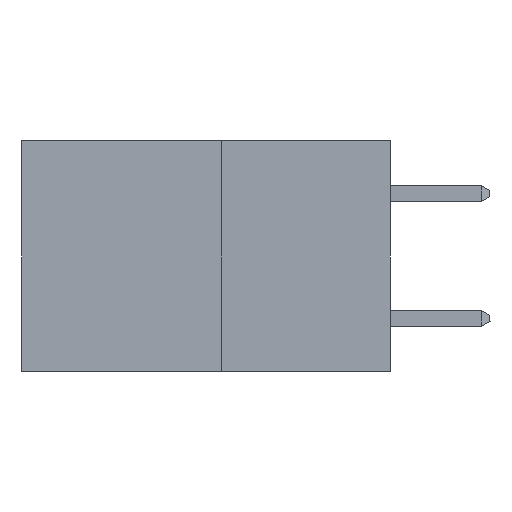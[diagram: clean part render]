
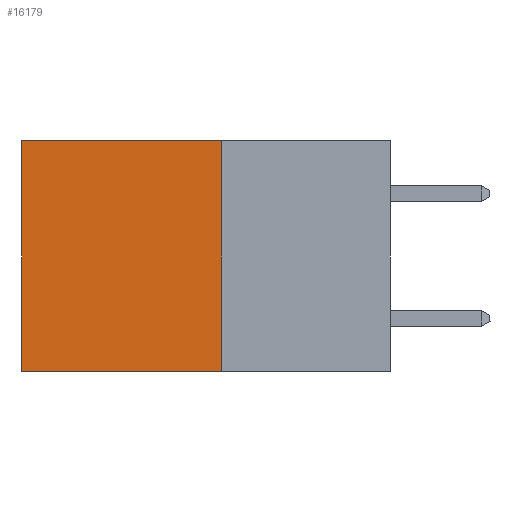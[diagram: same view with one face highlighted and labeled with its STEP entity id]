
A CAD part, left-side view. The second image highlights one B-rep face of the part: STEP entity #16179.
In plain terms, the highlighted planar face has unit normal (-1, 0, 0).
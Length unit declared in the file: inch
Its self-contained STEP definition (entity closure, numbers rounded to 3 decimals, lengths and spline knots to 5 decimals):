
#181 = VERTEX_POINT ( 'NONE', #3201 ) ;
#995 = EDGE_LOOP ( 'NONE', ( #20365, #12897, #12182, #19189 ) ) ;
#2464 = LINE ( 'NONE', #17334, #7017 ) ;
#3201 = CARTESIAN_POINT ( 'NONE',  ( 0.277, 0.59, -0.37 ) ) ;
#3960 = VECTOR ( 'NONE', #12207, 39.37008 ) ;
#4144 = EDGE_CURVE ( 'NONE', #6249, #20499, #17325, .T. ) ;
#6064 = EDGE_CURVE ( 'NONE', #19152, #181, #20495, .T. ) ;
#6249 = VERTEX_POINT ( 'NONE', #13793 ) ;
#7017 = VECTOR ( 'NONE', #7375, 39.37008 ) ;
#7375 = DIRECTION ( 'NONE',  ( 0., 0., -1. ) ) ;
#7764 = CARTESIAN_POINT ( 'NONE',  ( 0.277, 0.59, 0. ) ) ;
#8077 = DIRECTION ( 'NONE',  ( 0., 0., -1. ) ) ;
#8523 = VECTOR ( 'NONE', #9554, 39.37008 ) ;
#9554 = DIRECTION ( 'NONE',  ( 0., 0., -1. ) ) ;
#10197 = FACE_OUTER_BOUND ( 'NONE', #995, .T. ) ;
#11511 = CARTESIAN_POINT ( 'NONE',  ( 0.277, 0.27, 0. ) ) ;
#12017 = AXIS2_PLACEMENT_3D ( 'NONE', #14697, #18030, #8077 ) ;
#12182 = ORIENTED_EDGE ( 'NONE', *, *, #18640, .F. ) ;
#12207 = DIRECTION ( 'NONE',  ( 0., 1., 0. ) ) ;
#12239 = VECTOR ( 'NONE', #16330, 39.37008 ) ;
#12394 = LINE ( 'NONE', #19468, #8523 ) ;
#12897 = ORIENTED_EDGE ( 'NONE', *, *, #6064, .F. ) ;
#13793 = CARTESIAN_POINT ( 'NONE',  ( 0.277, 0.27, 0. ) ) ;
#14697 = CARTESIAN_POINT ( 'NONE',  ( 0.277, 0.27, -0.37 ) ) ;
#16179 = ADVANCED_FACE ( 'NONE', ( #10197 ), #16317, .F. ) ;
#16317 = PLANE ( 'NONE',  #12017 ) ;
#16330 = DIRECTION ( 'NONE',  ( 0., 1., 0. ) ) ;
#16399 = CARTESIAN_POINT ( 'NONE',  ( 0.277, 0.27, -0.37 ) ) ;
#17325 = LINE ( 'NONE', #11511, #3960 ) ;
#17334 = CARTESIAN_POINT ( 'NONE',  ( 0.277, 0.59, -0.37 ) ) ;
#17823 = EDGE_CURVE ( 'NONE', #20499, #181, #2464, .T. ) ;
#18030 = DIRECTION ( 'NONE',  ( 1., 0., 0. ) ) ;
#18640 = EDGE_CURVE ( 'NONE', #6249, #19152, #12394, .T. ) ;
#19152 = VERTEX_POINT ( 'NONE', #20873 ) ;
#19189 = ORIENTED_EDGE ( 'NONE', *, *, #4144, .T. ) ;
#19468 = CARTESIAN_POINT ( 'NONE',  ( 0.277, 0.27, -0.37 ) ) ;
#20365 = ORIENTED_EDGE ( 'NONE', *, *, #17823, .T. ) ;
#20495 = LINE ( 'NONE', #16399, #12239 ) ;
#20499 = VERTEX_POINT ( 'NONE', #7764 ) ;
#20873 = CARTESIAN_POINT ( 'NONE',  ( 0.277, 0.27, -0.37 ) ) ;
